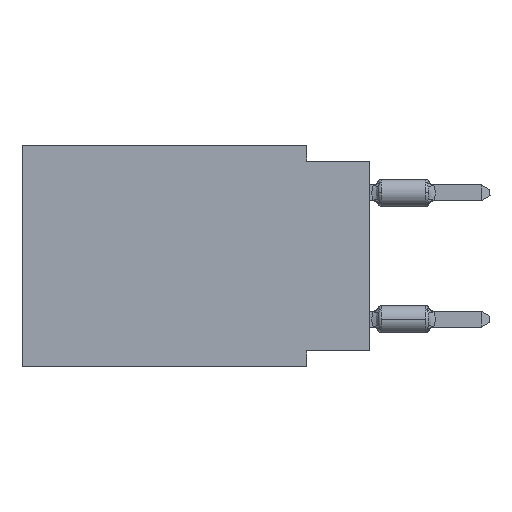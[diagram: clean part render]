
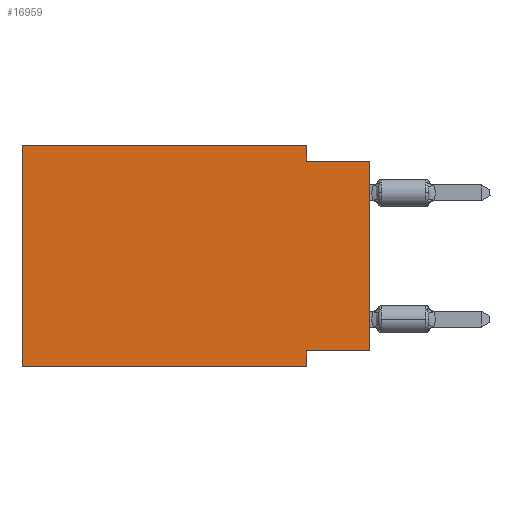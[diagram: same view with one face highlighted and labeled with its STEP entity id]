
A CAD part, left-side view. The second image highlights one B-rep face of the part: STEP entity #16959.
In plain terms, the highlighted planar face has unit normal (-1, 0, 0).
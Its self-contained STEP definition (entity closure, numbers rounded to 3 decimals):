
#510 = CARTESIAN_POINT ( 'NONE',  ( 0., 0., -0.635 ) ) ;
#2656 = EDGE_CURVE ( 'NONE', #12678, #33692, #30095, .T. ) ;
#3055 = DIRECTION ( 'NONE',  ( 0., 1., 0. ) ) ;
#3660 = ORIENTED_EDGE ( 'NONE', *, *, #44858, .F. ) ;
#4011 = PLANE ( 'NONE',  #19056 ) ;
#4307 = VECTOR ( 'NONE', #34440, 1000. ) ;
#5266 = DIRECTION ( 'NONE',  ( 0., 0., -1. ) ) ;
#5372 = CARTESIAN_POINT ( 'NONE',  ( 0., 13.97, -8.89 ) ) ;
#5946 = ORIENTED_EDGE ( 'NONE', *, *, #2656, .F. ) ;
#6087 = DIRECTION ( 'NONE',  ( 0., 0., 1. ) ) ;
#6770 = ORIENTED_EDGE ( 'NONE', *, *, #9113, .T. ) ;
#7062 = ORIENTED_EDGE ( 'NONE', *, *, #39032, .T. ) ;
#8358 = CARTESIAN_POINT ( 'NONE',  ( 0., 2.54, -8.255 ) ) ;
#8996 = CARTESIAN_POINT ( 'NONE',  ( 0., 0., -0.635 ) ) ;
#9113 = EDGE_CURVE ( 'NONE', #36828, #24453, #34239, .T. ) ;
#9735 = VERTEX_POINT ( 'NONE', #13066 ) ;
#11766 = LINE ( 'NONE', #37678, #31919 ) ;
#12678 = VERTEX_POINT ( 'NONE', #43939 ) ;
#13066 = CARTESIAN_POINT ( 'NONE',  ( 0., 0., -8.255 ) ) ;
#13070 = LINE ( 'NONE', #15969, #4307 ) ;
#15341 = ORIENTED_EDGE ( 'NONE', *, *, #35619, .F. ) ;
#15512 = ORIENTED_EDGE ( 'NONE', *, *, #31339, .F. ) ;
#15969 = CARTESIAN_POINT ( 'NONE',  ( 0., 0., 0. ) ) ;
#16959 = ADVANCED_FACE ( 'NONE', ( #33974 ), #4011, .F. ) ;
#18177 = CARTESIAN_POINT ( 'NONE',  ( 0., 2.54, -0.635 ) ) ;
#18402 = CARTESIAN_POINT ( 'NONE',  ( 0., 2.54, 0. ) ) ;
#18404 = VERTEX_POINT ( 'NONE', #8358 ) ;
#18632 = CARTESIAN_POINT ( 'NONE',  ( 0., 13.97, -8.89 ) ) ;
#19056 = AXIS2_PLACEMENT_3D ( 'NONE', #19339, #30385, #45731 ) ;
#19150 = VECTOR ( 'NONE', #44322, 1000. ) ;
#19339 = CARTESIAN_POINT ( 'NONE',  ( 0., 13.97, 0. ) ) ;
#20033 = VECTOR ( 'NONE', #43967, 1000. ) ;
#20947 = CARTESIAN_POINT ( 'NONE',  ( 0., 2.54, -8.89 ) ) ;
#23864 = CARTESIAN_POINT ( 'NONE',  ( 0., 13.97, 0. ) ) ;
#24453 = VERTEX_POINT ( 'NONE', #40036 ) ;
#27474 = LINE ( 'NONE', #23864, #37866 ) ;
#27754 = EDGE_CURVE ( 'NONE', #33692, #46085, #11766, .T. ) ;
#28556 = ORIENTED_EDGE ( 'NONE', *, *, #27754, .F. ) ;
#28681 = VERTEX_POINT ( 'NONE', #8996 ) ;
#29857 = CARTESIAN_POINT ( 'NONE',  ( 0., 13.97, 0. ) ) ;
#30095 = LINE ( 'NONE', #29857, #34927 ) ;
#30385 = DIRECTION ( 'NONE',  ( 1., 0., 0. ) ) ;
#31339 = EDGE_CURVE ( 'NONE', #18404, #24453, #39194, .T. ) ;
#31919 = VECTOR ( 'NONE', #5266, 1000. ) ;
#32712 = EDGE_CURVE ( 'NONE', #46085, #28681, #33883, .T. ) ;
#33692 = VERTEX_POINT ( 'NONE', #18402 ) ;
#33883 = LINE ( 'NONE', #510, #20033 ) ;
#33974 = FACE_OUTER_BOUND ( 'NONE', #42496, .T. ) ;
#34239 = LINE ( 'NONE', #18632, #19150 ) ;
#34440 = DIRECTION ( 'NONE',  ( 0., 0., 1. ) ) ;
#34927 = VECTOR ( 'NONE', #44492, 1000. ) ;
#35619 = EDGE_CURVE ( 'NONE', #36828, #12678, #27474, .T. ) ;
#35828 = DIRECTION ( 'NONE',  ( 0., 0., -1. ) ) ;
#36828 = VERTEX_POINT ( 'NONE', #5372 ) ;
#37678 = CARTESIAN_POINT ( 'NONE',  ( 0., 2.54, 0. ) ) ;
#37866 = VECTOR ( 'NONE', #6087, 1000. ) ;
#39032 = EDGE_CURVE ( 'NONE', #9735, #28681, #13070, .T. ) ;
#39194 = LINE ( 'NONE', #20947, #41445 ) ;
#40036 = CARTESIAN_POINT ( 'NONE',  ( 0., 2.54, -8.89 ) ) ;
#40265 = CARTESIAN_POINT ( 'NONE',  ( 0., 0., -8.255 ) ) ;
#41445 = VECTOR ( 'NONE', #35828, 1000. ) ;
#42496 = EDGE_LOOP ( 'NONE', ( #7062, #46520, #28556, #5946, #15341, #6770, #15512, #3660 ) ) ;
#43939 = CARTESIAN_POINT ( 'NONE',  ( 0., 13.97, 0. ) ) ;
#43967 = DIRECTION ( 'NONE',  ( 0., -1., 0. ) ) ;
#44322 = DIRECTION ( 'NONE',  ( 0., -1., 0. ) ) ;
#44492 = DIRECTION ( 'NONE',  ( 0., -1., 0. ) ) ;
#44858 = EDGE_CURVE ( 'NONE', #9735, #18404, #47004, .T. ) ;
#44948 = VECTOR ( 'NONE', #3055, 1000. ) ;
#45731 = DIRECTION ( 'NONE',  ( 0., 0., -1. ) ) ;
#46085 = VERTEX_POINT ( 'NONE', #18177 ) ;
#46520 = ORIENTED_EDGE ( 'NONE', *, *, #32712, .F. ) ;
#47004 = LINE ( 'NONE', #40265, #44948 ) ;
